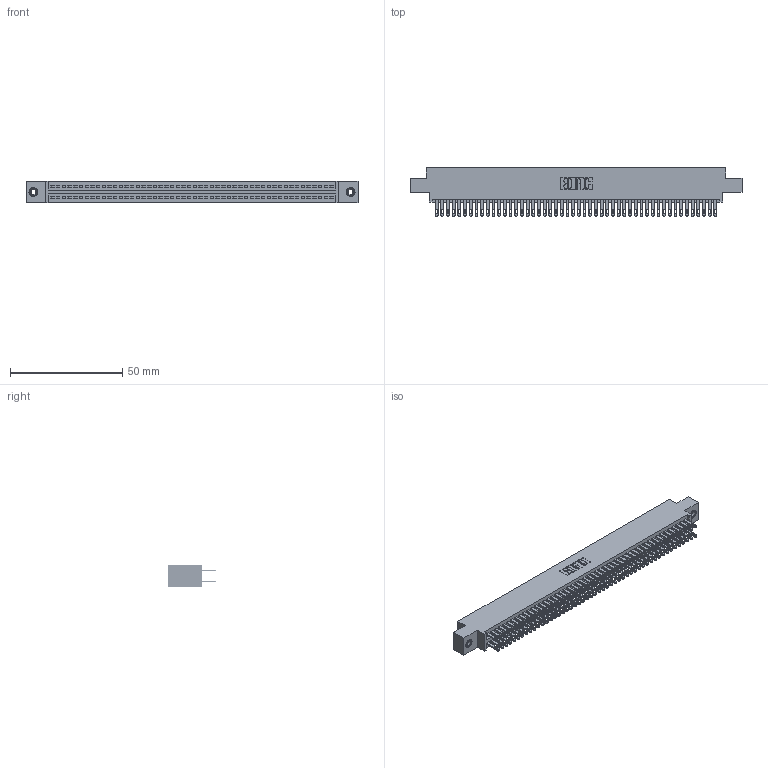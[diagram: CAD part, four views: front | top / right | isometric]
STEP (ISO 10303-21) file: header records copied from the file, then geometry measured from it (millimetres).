
FILE_DESCRIPTION (( 'STEP AP203' ), '1' );
FILE_NAME ('345-100-500-808.STEP', '2019-11-02T14:01:20', ( '' ), ( '' ), 'SwSTEP 2.0', 'SolidWorks 2016', '' );
FILE_SCHEMA (( 'CONFIG_CONTROL_DESIGN' ));
Length unit declared in the file: inch
Products named in the file (4): 345-250-001_345-250-003-102; 345-100-500-808; 345-292-001_345-293-100; 345 Part_0.170 Offset - 0.156 Dia-TI
Assembly tree (103 placements, depth 2):
  345-100-500-808
    345 Part_0.170 Offset - 0.156 Dia-TI
    345-292-001_345-293-100  x100
    345-250-001_345-250-003-102  x2
Bounding box: 148.21 x 21.51 x 9.4 mm (x, y, z)
Volume: 14657.1 mm3; surface area: 22997.5 mm2
Topology: 103 solids, 103 shells, 4790 faces, 14589 edges, 9718 vertices
Faces by surface type: plane 2816, cylinder 1958, cone 12, torus 4
Entity records: 39402 total; most frequent: CARTESIAN_POINT 6579, ORIENTED_EDGE 6506, DIRECTION 5819, EDGE_CURVE 3253, VECTOR 2897, LINE 2897, VERTEX_POINT 2164, AXIS2_PLACEMENT_3D 1461
